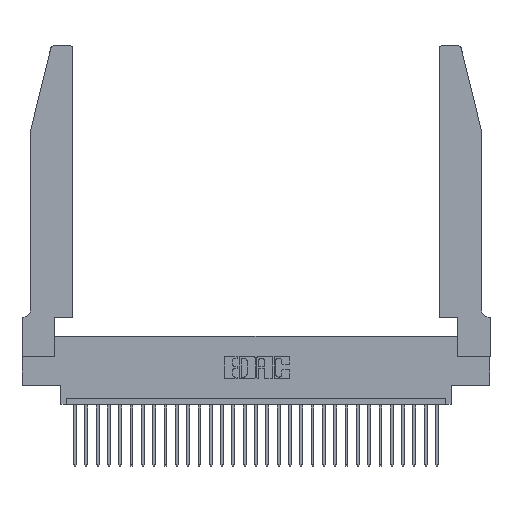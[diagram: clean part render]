
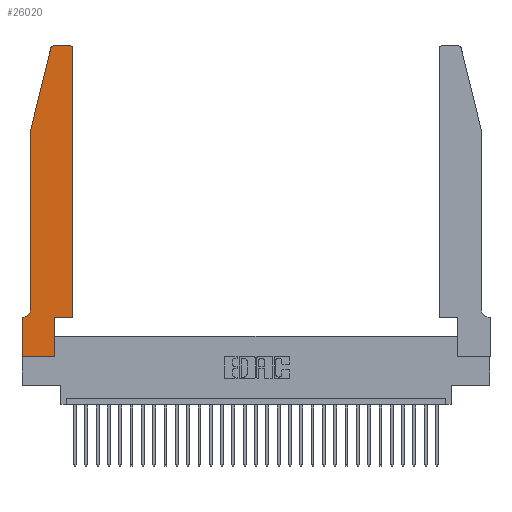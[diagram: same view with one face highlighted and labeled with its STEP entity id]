
A CAD part, top view. The second image highlights one B-rep face of the part: STEP entity #26020.
In plain terms, the highlighted planar face has unit normal (0, 0, 1).
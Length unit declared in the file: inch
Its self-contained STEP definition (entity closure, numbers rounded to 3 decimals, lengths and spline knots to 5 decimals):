
#378 = VERTEX_POINT ( 'NONE', #4674 ) ;
#1319 = EDGE_CURVE ( 'NONE', #13838, #29600, #5898, .T. ) ;
#1630 = DIRECTION ( 'NONE',  ( 0., -1., 0. ) ) ;
#1966 = DIRECTION ( 'NONE',  ( 0., 1., 0. ) ) ;
#2370 = ORIENTED_EDGE ( 'NONE', *, *, #30705, .T. ) ;
#2422 = ORIENTED_EDGE ( 'NONE', *, *, #18488, .T. ) ;
#2908 = DIRECTION ( 'NONE',  ( 1., 0., 0. ) ) ;
#3549 = ORIENTED_EDGE ( 'NONE', *, *, #16227, .T. ) ;
#3635 = DIRECTION ( 'NONE',  ( 0., -1., 0. ) ) ;
#3813 = VERTEX_POINT ( 'NONE', #20846 ) ;
#4674 = CARTESIAN_POINT ( 'NONE',  ( 0.0055, 0.35, 0.37 ) ) ;
#5139 = VECTOR ( 'NONE', #11219, 39.37008 ) ;
#5164 = CARTESIAN_POINT ( 'NONE',  ( 0., 0.35, 0.37 ) ) ;
#5326 = VECTOR ( 'NONE', #1630, 39.37008 ) ;
#5768 = CARTESIAN_POINT ( 'NONE',  ( 0.4205, 2.75, 0.37 ) ) ;
#5898 = LINE ( 'NONE', #16115, #13688 ) ;
#6571 = DIRECTION ( 'NONE',  ( 0., 0., 1. ) ) ;
#6619 = CARTESIAN_POINT ( 'NONE',  ( 0.0755, 2., 0.37 ) ) ;
#7596 = VECTOR ( 'NONE', #17691, 39.37008 ) ;
#7880 = CIRCLE ( 'NONE', #16105, 0.03 ) ;
#8140 = CARTESIAN_POINT ( 'NONE',  ( 0.2865, 0.35, 0.37 ) ) ;
#8401 = FACE_OUTER_BOUND ( 'NONE', #23932, .T. ) ;
#8868 = ORIENTED_EDGE ( 'NONE', *, *, #25126, .T. ) ;
#9364 = VERTEX_POINT ( 'NONE', #17583 ) ;
#10171 = DIRECTION ( 'NONE',  ( 0., 0., 1. ) ) ;
#10359 = VECTOR ( 'NONE', #10621, 39.37008 ) ;
#10621 = DIRECTION ( 'NONE',  ( 0., 1., 0. ) ) ;
#10829 = CARTESIAN_POINT ( 'NONE',  ( 0.2865, 0.35, 0.37 ) ) ;
#11219 = DIRECTION ( 'NONE',  ( 1., 0., 0. ) ) ;
#11344 = EDGE_CURVE ( 'NONE', #378, #15692, #28971, .T. ) ;
#11803 = LINE ( 'NONE', #27681, #22623 ) ;
#12865 = VERTEX_POINT ( 'NONE', #19971 ) ;
#13039 = AXIS2_PLACEMENT_3D ( 'NONE', #23755, #21117, #13756 ) ;
#13375 = CARTESIAN_POINT ( 'NONE',  ( 0.0055, 0.42, 0.37 ) ) ;
#13623 = DIRECTION ( 'NONE',  ( 1., 0., 0. ) ) ;
#13626 = EDGE_CURVE ( 'NONE', #16185, #9364, #26733, .T. ) ;
#13642 = CIRCLE ( 'NONE', #27392, 0.03 ) ;
#13688 = VECTOR ( 'NONE', #1966, 39.37008 ) ;
#13739 = LINE ( 'NONE', #6619, #16760 ) ;
#13756 = DIRECTION ( 'NONE',  ( 1., 0., 0. ) ) ;
#13838 = VERTEX_POINT ( 'NONE', #30489 ) ;
#14379 = CARTESIAN_POINT ( 'NONE',  ( 0.4505, 2.72, 0.37 ) ) ;
#14430 = ORIENTED_EDGE ( 'NONE', *, *, #11344, .T. ) ;
#15272 = CARTESIAN_POINT ( 'NONE',  ( 0., 0., 0.37 ) ) ;
#15336 = ORIENTED_EDGE ( 'NONE', *, *, #17472, .T. ) ;
#15521 = CIRCLE ( 'NONE', #20767, 0.07 ) ;
#15619 = CARTESIAN_POINT ( 'NONE',  ( 0.284, 2.72, 0.37 ) ) ;
#15692 = VERTEX_POINT ( 'NONE', #5164 ) ;
#15847 = VERTEX_POINT ( 'NONE', #21846 ) ;
#15966 = ORIENTED_EDGE ( 'NONE', *, *, #17935, .T. ) ;
#16105 = AXIS2_PLACEMENT_3D ( 'NONE', #24558, #10171, #2908 ) ;
#16115 = CARTESIAN_POINT ( 'NONE',  ( 0.4505, 0.35, 0.37 ) ) ;
#16183 = VECTOR ( 'NONE', #29983, 39.37008 ) ;
#16185 = VERTEX_POINT ( 'NONE', #5768 ) ;
#16227 = EDGE_CURVE ( 'NONE', #25049, #30413, #13739, .T. ) ;
#16760 = VECTOR ( 'NONE', #28157, 39.37008 ) ;
#17472 = EDGE_CURVE ( 'NONE', #20894, #13838, #23480, .T. ) ;
#17583 = CARTESIAN_POINT ( 'NONE',  ( 0.284, 2.75, 0.37 ) ) ;
#17691 = DIRECTION ( 'NONE',  ( -1., 0., 0. ) ) ;
#17824 = LINE ( 'NONE', #10829, #10359 ) ;
#17935 = EDGE_CURVE ( 'NONE', #12865, #378, #15521, .T. ) ;
#18304 = DIRECTION ( 'NONE',  ( 1., 0., 0. ) ) ;
#18488 = EDGE_CURVE ( 'NONE', #9364, #25049, #13642, .T. ) ;
#18692 = LINE ( 'NONE', #15272, #26595 ) ;
#18945 = ORIENTED_EDGE ( 'NONE', *, *, #13626, .T. ) ;
#19971 = CARTESIAN_POINT ( 'NONE',  ( 0.0755, 0.42, 0.37 ) ) ;
#20646 = ORIENTED_EDGE ( 'NONE', *, *, #23581, .T. ) ;
#20767 = AXIS2_PLACEMENT_3D ( 'NONE', #13375, #23174, #27685 ) ;
#20846 = CARTESIAN_POINT ( 'NONE',  ( 0.2865, 0., 0.37 ) ) ;
#20894 = VERTEX_POINT ( 'NONE', #8140 ) ;
#21117 = DIRECTION ( 'NONE',  ( 0., 0., 1. ) ) ;
#21846 = CARTESIAN_POINT ( 'NONE',  ( 0., 0., 0.37 ) ) ;
#22548 = CARTESIAN_POINT ( 'NONE',  ( 0.2605, 2.75, 0.37 ) ) ;
#22623 = VECTOR ( 'NONE', #3635, 39.37008 ) ;
#23174 = DIRECTION ( 'NONE',  ( 0., 0., -1. ) ) ;
#23480 = LINE ( 'NONE', #25504, #5139 ) ;
#23581 = EDGE_CURVE ( 'NONE', #15692, #15847, #27031, .T. ) ;
#23652 = PLANE ( 'NONE',  #13039 ) ;
#23755 = CARTESIAN_POINT ( 'NONE',  ( 0., 0.35, 0.37 ) ) ;
#23932 = EDGE_LOOP ( 'NONE', ( #18945, #2422, #3549, #26017, #15966, #14430, #20646, #8868, #2370, #15336, #29686, #29215 ) ) ;
#24459 = CARTESIAN_POINT ( 'NONE',  ( 0.0755, 0.35, 0.37 ) ) ;
#24558 = CARTESIAN_POINT ( 'NONE',  ( 0.4205, 2.72, 0.37 ) ) ;
#25049 = VERTEX_POINT ( 'NONE', #27362 ) ;
#25126 = EDGE_CURVE ( 'NONE', #15847, #3813, #18692, .T. ) ;
#25187 = EDGE_CURVE ( 'NONE', #30413, #12865, #11803, .T. ) ;
#25504 = CARTESIAN_POINT ( 'NONE',  ( 0.4505, 0.35, 0.37 ) ) ;
#26017 = ORIENTED_EDGE ( 'NONE', *, *, #25187, .T. ) ;
#26020 = ADVANCED_FACE ( 'NONE', ( #8401 ), #23652, .T. ) ;
#26487 = CARTESIAN_POINT ( 'NONE',  ( 0.0755, 2., 0.37 ) ) ;
#26595 = VECTOR ( 'NONE', #18304, 39.37008 ) ;
#26733 = LINE ( 'NONE', #22548, #7596 ) ;
#27031 = LINE ( 'NONE', #30273, #5326 ) ;
#27362 = CARTESIAN_POINT ( 'NONE',  ( 0.25487, 2.72718, 0.37 ) ) ;
#27392 = AXIS2_PLACEMENT_3D ( 'NONE', #15619, #6571, #13623 ) ;
#27681 = CARTESIAN_POINT ( 'NONE',  ( 0.0755, 2., 0.37 ) ) ;
#27685 = DIRECTION ( 'NONE',  ( -1., 0., 0. ) ) ;
#28157 = DIRECTION ( 'NONE',  ( -0.239, -0.971, 0. ) ) ;
#28569 = EDGE_CURVE ( 'NONE', #29600, #16185, #7880, .T. ) ;
#28971 = LINE ( 'NONE', #24459, #16183 ) ;
#29215 = ORIENTED_EDGE ( 'NONE', *, *, #28569, .T. ) ;
#29600 = VERTEX_POINT ( 'NONE', #14379 ) ;
#29686 = ORIENTED_EDGE ( 'NONE', *, *, #1319, .T. ) ;
#29983 = DIRECTION ( 'NONE',  ( -1., 0., 0. ) ) ;
#30273 = CARTESIAN_POINT ( 'NONE',  ( 0., 0., 0.37 ) ) ;
#30413 = VERTEX_POINT ( 'NONE', #26487 ) ;
#30489 = CARTESIAN_POINT ( 'NONE',  ( 0.4505, 0.35, 0.37 ) ) ;
#30705 = EDGE_CURVE ( 'NONE', #3813, #20894, #17824, .T. ) ;
